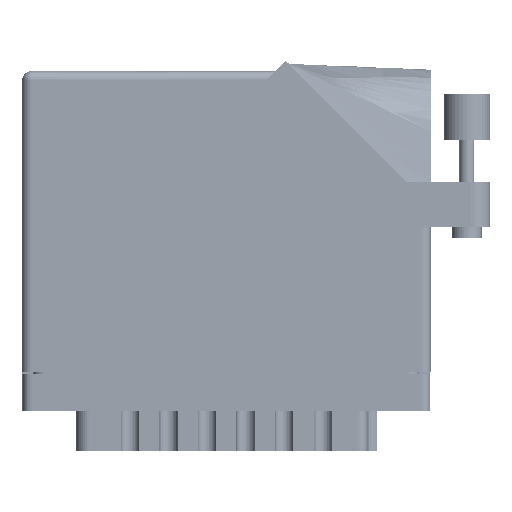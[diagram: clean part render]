
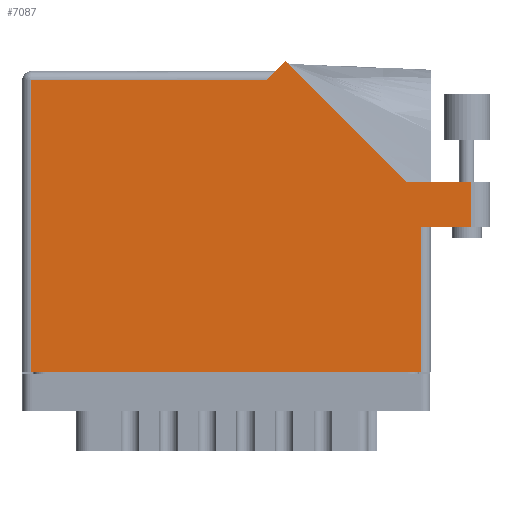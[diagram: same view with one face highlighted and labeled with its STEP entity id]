
A CAD part, front view. The second image highlights one B-rep face of the part: STEP entity #7087.
In plain terms, the highlighted face is planar.
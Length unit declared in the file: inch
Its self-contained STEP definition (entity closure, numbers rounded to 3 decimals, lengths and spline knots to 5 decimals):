
#393 = CARTESIAN_POINT ( 'NONE',  ( 0.062, 0., 0. ) ) ;
#467 = DIRECTION ( 'NONE',  ( 1., 0., 0. ) ) ;
#721 = EDGE_CURVE ( 'NONE', #49251, #86594, #2766, .T. ) ;
#979 = EDGE_LOOP ( 'NONE', ( #13501, #84717, #49360, #24715, #36366, #66405, #57879, #13918, #50696 ) ) ;
#2416 = VECTOR ( 'NONE', #53708, 39.37008 ) ;
#2766 = LINE ( 'NONE', #63422, #8481 ) ;
#3306 = PLANE ( 'NONE',  #24518 ) ;
#3461 = CARTESIAN_POINT ( 'NONE',  ( 3.03, 1.287, 0. ) ) ;
#4311 = VECTOR ( 'NONE', #26928, 39.37008 ) ;
#7087 = ADVANCED_FACE ( 'NONE', ( #42142 ), #3306, .F. ) ;
#7356 = DIRECTION ( 'NONE',  ( 0., 1., 0. ) ) ;
#8481 = VECTOR ( 'NONE', #7356, 39.37008 ) ;
#8575 = VECTOR ( 'NONE', #69476, 39.37008 ) ;
#9303 = VERTEX_POINT ( 'NONE', #32906 ) ;
#11815 = CARTESIAN_POINT ( 'NONE',  ( 1.643, 1.968, 0. ) ) ;
#13501 = ORIENTED_EDGE ( 'NONE', *, *, #42967, .T. ) ;
#13918 = ORIENTED_EDGE ( 'NONE', *, *, #81593, .T. ) ;
#17415 = VERTEX_POINT ( 'NONE', #3461 ) ;
#17594 = VECTOR ( 'NONE', #467, 39.37008 ) ;
#19679 = CARTESIAN_POINT ( 'NONE',  ( 3.03, 1.287, 0. ) ) ;
#23895 = LINE ( 'NONE', #27062, #87988 ) ;
#24183 = VECTOR ( 'NONE', #72712, 39.37008 ) ;
#24518 = AXIS2_PLACEMENT_3D ( 'NONE', #45888, #31376, #82224 ) ;
#24715 = ORIENTED_EDGE ( 'NONE', *, *, #92661, .T. ) ;
#26928 = DIRECTION ( 'NONE',  ( 0., 1., 0. ) ) ;
#27062 = CARTESIAN_POINT ( 'NONE',  ( 1.705, 2.03, 0. ) ) ;
#27985 = LINE ( 'NONE', #19679, #4311 ) ;
#31064 = LINE ( 'NONE', #79375, #17594 ) ;
#31376 = DIRECTION ( 'NONE',  ( 0., 0., -1. ) ) ;
#31572 = VERTEX_POINT ( 'NONE', #88791 ) ;
#32906 = CARTESIAN_POINT ( 'NONE',  ( 0.062, 1.968, 0. ) ) ;
#33046 = CARTESIAN_POINT ( 'NONE',  ( 3.03, 0.98, 0. ) ) ;
#36366 = ORIENTED_EDGE ( 'NONE', *, *, #89856, .T. ) ;
#40984 = VERTEX_POINT ( 'NONE', #86689 ) ;
#42142 = FACE_OUTER_BOUND ( 'NONE', #979, .T. ) ;
#42967 = EDGE_CURVE ( 'NONE', #86594, #43407, #78173, .T. ) ;
#43407 = VERTEX_POINT ( 'NONE', #33046 ) ;
#44103 = LINE ( 'NONE', #62152, #2416 ) ;
#45888 = CARTESIAN_POINT ( 'NONE',  ( 0., 2.03, 0. ) ) ;
#46685 = LINE ( 'NONE', #79903, #81403 ) ;
#49251 = VERTEX_POINT ( 'NONE', #75834 ) ;
#49360 = ORIENTED_EDGE ( 'NONE', *, *, #75934, .T. ) ;
#50696 = ORIENTED_EDGE ( 'NONE', *, *, #721, .T. ) ;
#53708 = DIRECTION ( 'NONE',  ( -1., 0., 0. ) ) ;
#55749 = DIRECTION ( 'NONE',  ( -0.707, -0.707, 0. ) ) ;
#56043 = DIRECTION ( 'NONE',  ( -0.707, 0.707, 0. ) ) ;
#57879 = ORIENTED_EDGE ( 'NONE', *, *, #88118, .T. ) ;
#59259 = DIRECTION ( 'NONE',  ( 0., -1., 0. ) ) ;
#62152 = CARTESIAN_POINT ( 'NONE',  ( 3.155, 1.287, 0. ) ) ;
#62670 = LINE ( 'NONE', #83548, #8575 ) ;
#63422 = CARTESIAN_POINT ( 'NONE',  ( 2.693, 0.98, 0. ) ) ;
#63659 = EDGE_CURVE ( 'NONE', #43407, #17415, #27985, .T. ) ;
#65813 = CARTESIAN_POINT ( 'NONE',  ( 2.755, 0.98, 0. ) ) ;
#66405 = ORIENTED_EDGE ( 'NONE', *, *, #93091, .T. ) ;
#69476 = DIRECTION ( 'NONE',  ( -1., 0., 0. ) ) ;
#72712 = DIRECTION ( 'NONE',  ( 1., 0., 0. ) ) ;
#75834 = CARTESIAN_POINT ( 'NONE',  ( 2.693, 0., 0. ) ) ;
#75934 = EDGE_CURVE ( 'NONE', #17415, #40984, #44103, .T. ) ;
#76198 = VECTOR ( 'NONE', #56043, 39.37008 ) ;
#77320 = CARTESIAN_POINT ( 'NONE',  ( 2.58942, 1.287, 0. ) ) ;
#78173 = LINE ( 'NONE', #65813, #24183 ) ;
#79375 = CARTESIAN_POINT ( 'NONE',  ( 0., 0., 0. ) ) ;
#79903 = CARTESIAN_POINT ( 'NONE',  ( 0.062, 0., 0. ) ) ;
#81403 = VECTOR ( 'NONE', #59259, 39.37008 ) ;
#81593 = EDGE_CURVE ( 'NONE', #83329, #49251, #31064, .T. ) ;
#82224 = DIRECTION ( 'NONE',  ( -1., 0., 0. ) ) ;
#83329 = VERTEX_POINT ( 'NONE', #393 ) ;
#83548 = CARTESIAN_POINT ( 'NONE',  ( 0., 1.968, 0. ) ) ;
#84717 = ORIENTED_EDGE ( 'NONE', *, *, #63659, .T. ) ;
#85875 = VERTEX_POINT ( 'NONE', #11815 ) ;
#86594 = VERTEX_POINT ( 'NONE', #91140 ) ;
#86689 = CARTESIAN_POINT ( 'NONE',  ( 2.58942, 1.287, 0. ) ) ;
#87988 = VECTOR ( 'NONE', #55749, 39.37008 ) ;
#88118 = EDGE_CURVE ( 'NONE', #9303, #83329, #46685, .T. ) ;
#88791 = CARTESIAN_POINT ( 'NONE',  ( 1.77571, 2.10071, 0. ) ) ;
#89856 = EDGE_CURVE ( 'NONE', #31572, #85875, #23895, .T. ) ;
#90769 = LINE ( 'NONE', #77320, #76198 ) ;
#91140 = CARTESIAN_POINT ( 'NONE',  ( 2.693, 0.98, 0. ) ) ;
#92661 = EDGE_CURVE ( 'NONE', #40984, #31572, #90769, .T. ) ;
#93091 = EDGE_CURVE ( 'NONE', #85875, #9303, #62670, .T. ) ;
